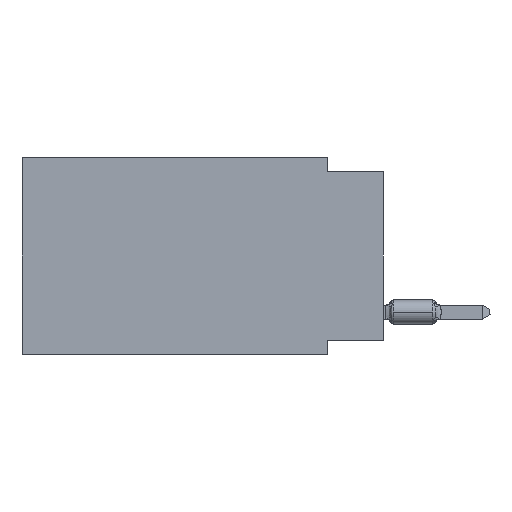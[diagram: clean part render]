
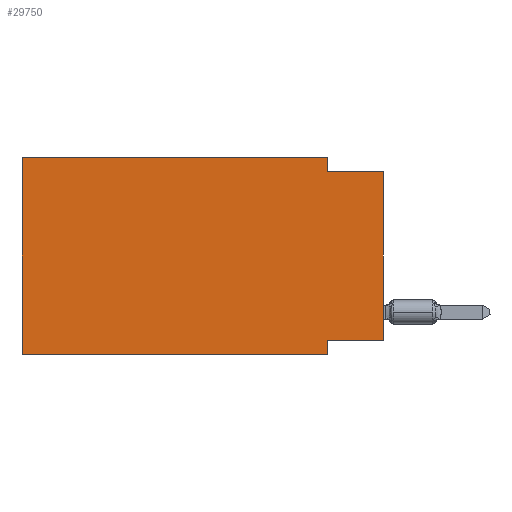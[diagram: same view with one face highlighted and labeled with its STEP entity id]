
A CAD part, left-side view. The second image highlights one B-rep face of the part: STEP entity #29750.
In plain terms, the highlighted planar face has unit normal (-1, 0, 0).
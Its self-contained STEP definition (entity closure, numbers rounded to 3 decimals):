
#5423 = ORIENTED_EDGE ( 'NONE', *, *, #101976, .F. ) ;
#5862 = VECTOR ( 'NONE', #49817, 1000. ) ;
#6010 = DIRECTION ( 'NONE',  ( 0., 0., -1. ) ) ;
#6023 = EDGE_CURVE ( 'NONE', #83618, #95001, #59683, .T. ) ;
#6032 = CARTESIAN_POINT ( 'NONE',  ( 0., 2.54, 0. ) ) ;
#7099 = VECTOR ( 'NONE', #40936, 1000. ) ;
#8296 = CARTESIAN_POINT ( 'NONE',  ( 0., 16.383, 0. ) ) ;
#12995 = DIRECTION ( 'NONE',  ( 0., 0., 1. ) ) ;
#16369 = CARTESIAN_POINT ( 'NONE',  ( 0., 2.54, -8.255 ) ) ;
#16662 = DIRECTION ( 'NONE',  ( 0., 1., 0. ) ) ;
#17033 = EDGE_CURVE ( 'NONE', #100633, #25041, #27556, .T. ) ;
#17173 = DIRECTION ( 'NONE',  ( 0., -1., 0. ) ) ;
#17806 = CARTESIAN_POINT ( 'NONE',  ( 0., 0., -8.255 ) ) ;
#19962 = CARTESIAN_POINT ( 'NONE',  ( 0., 16.383, 0. ) ) ;
#23659 = VECTOR ( 'NONE', #16662, 1000. ) ;
#25041 = VERTEX_POINT ( 'NONE', #94225 ) ;
#25904 = LINE ( 'NONE', #69437, #84433 ) ;
#27556 = LINE ( 'NONE', #19962, #102321 ) ;
#29731 = LINE ( 'NONE', #30863, #95881 ) ;
#29750 = ADVANCED_FACE ( 'NONE', ( #103511 ), #87810, .F. ) ;
#30429 = ORIENTED_EDGE ( 'NONE', *, *, #6023, .F. ) ;
#30863 = CARTESIAN_POINT ( 'NONE',  ( 0., 16.383, -8.89 ) ) ;
#31645 = CARTESIAN_POINT ( 'NONE',  ( 0., 16.383, 0. ) ) ;
#33771 = AXIS2_PLACEMENT_3D ( 'NONE', #8296, #42004, #6010 ) ;
#35665 = CARTESIAN_POINT ( 'NONE',  ( 0., 16.383, -8.89 ) ) ;
#36828 = DIRECTION ( 'NONE',  ( 0., -1., 0. ) ) ;
#40936 = DIRECTION ( 'NONE',  ( 0., 0., 1. ) ) ;
#41445 = DIRECTION ( 'NONE',  ( 0., 0., -1. ) ) ;
#42004 = DIRECTION ( 'NONE',  ( 1., 0., 0. ) ) ;
#44000 = EDGE_CURVE ( 'NONE', #44089, #100633, #104170, .T. ) ;
#44089 = VERTEX_POINT ( 'NONE', #35665 ) ;
#47559 = CARTESIAN_POINT ( 'NONE',  ( 0., 16.383, 0. ) ) ;
#48037 = VERTEX_POINT ( 'NONE', #78626 ) ;
#49817 = DIRECTION ( 'NONE',  ( 0., 0., -1. ) ) ;
#53261 = ORIENTED_EDGE ( 'NONE', *, *, #44000, .F. ) ;
#58862 = CARTESIAN_POINT ( 'NONE',  ( 0., 2.54, -0.635 ) ) ;
#59683 = LINE ( 'NONE', #95071, #5862 ) ;
#64551 = DIRECTION ( 'NONE',  ( 0., -1., 0. ) ) ;
#69437 = CARTESIAN_POINT ( 'NONE',  ( 0., 0., -0.635 ) ) ;
#70265 = EDGE_CURVE ( 'NONE', #75018, #48037, #25904, .T. ) ;
#71688 = ORIENTED_EDGE ( 'NONE', *, *, #75030, .F. ) ;
#73824 = CARTESIAN_POINT ( 'NONE',  ( 0., 2.54, -8.89 ) ) ;
#73998 = EDGE_CURVE ( 'NONE', #44089, #95001, #29731, .T. ) ;
#75018 = VERTEX_POINT ( 'NONE', #58862 ) ;
#75030 = EDGE_CURVE ( 'NONE', #25041, #75018, #85537, .T. ) ;
#75663 = LINE ( 'NONE', #84921, #113943 ) ;
#78626 = CARTESIAN_POINT ( 'NONE',  ( 0., 0., -0.635 ) ) ;
#78757 = LINE ( 'NONE', #17806, #23659 ) ;
#81278 = VECTOR ( 'NONE', #41445, 1000. ) ;
#83618 = VERTEX_POINT ( 'NONE', #16369 ) ;
#84433 = VECTOR ( 'NONE', #17173, 1000. ) ;
#84921 = CARTESIAN_POINT ( 'NONE',  ( 0., 0., 0. ) ) ;
#85537 = LINE ( 'NONE', #6032, #81278 ) ;
#85909 = EDGE_CURVE ( 'NONE', #96983, #48037, #75663, .T. ) ;
#87810 = PLANE ( 'NONE',  #33771 ) ;
#94225 = CARTESIAN_POINT ( 'NONE',  ( 0., 2.54, 0. ) ) ;
#94624 = EDGE_LOOP ( 'NONE', ( #106691, #101788, #71688, #107037, #53261, #109256, #30429, #5423 ) ) ;
#95001 = VERTEX_POINT ( 'NONE', #73824 ) ;
#95071 = CARTESIAN_POINT ( 'NONE',  ( 0., 2.54, -8.89 ) ) ;
#95881 = VECTOR ( 'NONE', #64551, 1000. ) ;
#96983 = VERTEX_POINT ( 'NONE', #103834 ) ;
#100633 = VERTEX_POINT ( 'NONE', #47559 ) ;
#101788 = ORIENTED_EDGE ( 'NONE', *, *, #70265, .F. ) ;
#101976 = EDGE_CURVE ( 'NONE', #96983, #83618, #78757, .T. ) ;
#102321 = VECTOR ( 'NONE', #36828, 1000. ) ;
#103511 = FACE_OUTER_BOUND ( 'NONE', #94624, .T. ) ;
#103834 = CARTESIAN_POINT ( 'NONE',  ( 0., 0., -8.255 ) ) ;
#104170 = LINE ( 'NONE', #31645, #7099 ) ;
#106691 = ORIENTED_EDGE ( 'NONE', *, *, #85909, .T. ) ;
#107037 = ORIENTED_EDGE ( 'NONE', *, *, #17033, .F. ) ;
#109256 = ORIENTED_EDGE ( 'NONE', *, *, #73998, .T. ) ;
#113943 = VECTOR ( 'NONE', #12995, 1000. ) ;
